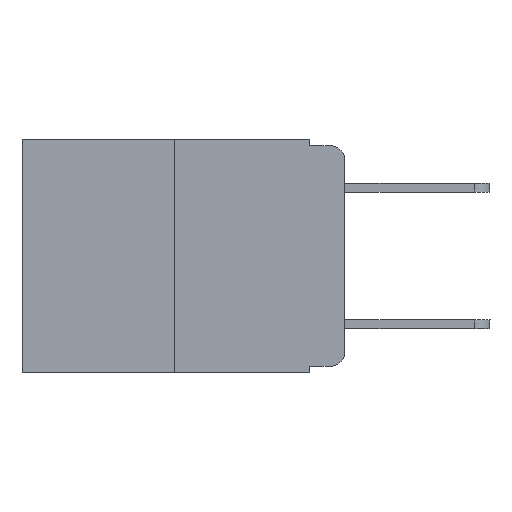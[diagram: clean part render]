
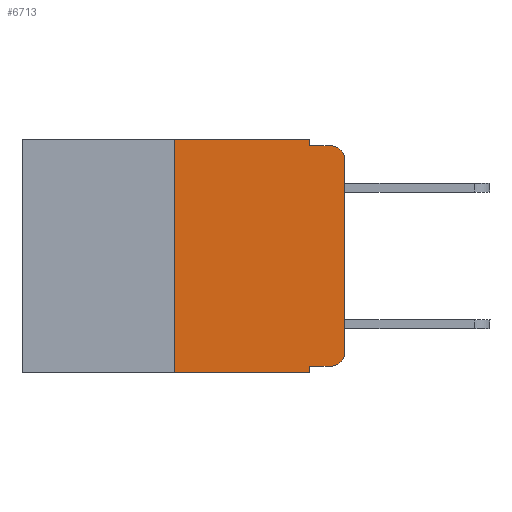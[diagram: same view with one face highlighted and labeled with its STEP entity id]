
A CAD part, left-side view. The second image highlights one B-rep face of the part: STEP entity #6713.
In plain terms, the highlighted planar face has unit normal (-1, 0, 0).
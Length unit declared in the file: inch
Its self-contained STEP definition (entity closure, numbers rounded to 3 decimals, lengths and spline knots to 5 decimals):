
#71 = CARTESIAN_POINT ( 'NONE',  ( 0., 0.051, -0.343 ) ) ;
#630 = VECTOR ( 'NONE', #10684, 39.37008 ) ;
#788 = LINE ( 'NONE', #16542, #19257 ) ;
#1191 = CARTESIAN_POINT ( 'NONE',  ( 0., 0.051, -0.333 ) ) ;
#1439 = EDGE_CURVE ( 'NONE', #18418, #3202, #11320, .T. ) ;
#2270 = VECTOR ( 'NONE', #10813, 39.37008 ) ;
#2386 = AXIS2_PLACEMENT_3D ( 'NONE', #9426, #15730, #13343 ) ;
#3202 = VERTEX_POINT ( 'NONE', #18172 ) ;
#3826 = ORIENTED_EDGE ( 'NONE', *, *, #18937, .F. ) ;
#4298 = CARTESIAN_POINT ( 'NONE',  ( 0., 0.473, 0. ) ) ;
#4370 = LINE ( 'NONE', #7563, #15542 ) ;
#4573 = EDGE_CURVE ( 'NONE', #18636, #16786, #20129, .T. ) ;
#4710 = EDGE_CURVE ( 'NONE', #7278, #18636, #17013, .T. ) ;
#5203 = ORIENTED_EDGE ( 'NONE', *, *, #12139, .F. ) ;
#5859 = DIRECTION ( 'NONE',  ( 0., 0., 1. ) ) ;
#6403 = DIRECTION ( 'NONE',  ( 0., 0., -1. ) ) ;
#6502 = CARTESIAN_POINT ( 'NONE',  ( 0., 0.051, 0. ) ) ;
#6581 = VECTOR ( 'NONE', #14652, 39.37008 ) ;
#6713 = ADVANCED_FACE ( 'NONE', ( #18058 ), #13406, .F. ) ;
#7006 = CARTESIAN_POINT ( 'NONE',  ( 0., 0.051, -0.01 ) ) ;
#7278 = VERTEX_POINT ( 'NONE', #19424 ) ;
#7444 = ORIENTED_EDGE ( 'NONE', *, *, #20322, .F. ) ;
#7563 = CARTESIAN_POINT ( 'NONE',  ( 0., 0.051, -0.333 ) ) ;
#7661 = CARTESIAN_POINT ( 'NONE',  ( 0., 0.02, -0.333 ) ) ;
#7866 = LINE ( 'NONE', #20189, #8780 ) ;
#7986 = CIRCLE ( 'NONE', #18227, 0.02 ) ;
#8211 = CARTESIAN_POINT ( 'NONE',  ( 0., 0., -0.03 ) ) ;
#8314 = EDGE_CURVE ( 'NONE', #15912, #20407, #7986, .T. ) ;
#8780 = VECTOR ( 'NONE', #20401, 39.37008 ) ;
#9102 = ORIENTED_EDGE ( 'NONE', *, *, #8314, .T. ) ;
#9426 = CARTESIAN_POINT ( 'NONE',  ( 0., 0.02, -0.313 ) ) ;
#9769 = DIRECTION ( 'NONE',  ( -1., 0., 0. ) ) ;
#10143 = CARTESIAN_POINT ( 'NONE',  ( 0., 0.25, 0. ) ) ;
#10561 = DIRECTION ( 'NONE',  ( 0., 0., -1. ) ) ;
#10659 = VECTOR ( 'NONE', #6403, 39.37008 ) ;
#10684 = DIRECTION ( 'NONE',  ( 0., 0., 1. ) ) ;
#10779 = ORIENTED_EDGE ( 'NONE', *, *, #16261, .T. ) ;
#10813 = DIRECTION ( 'NONE',  ( 0., -1., 0. ) ) ;
#10919 = LINE ( 'NONE', #12371, #14381 ) ;
#11187 = DIRECTION ( 'NONE',  ( 0., 0., -1. ) ) ;
#11320 = CIRCLE ( 'NONE', #2386, 0.02 ) ;
#11472 = CARTESIAN_POINT ( 'NONE',  ( 0., 0.051, 0. ) ) ;
#11646 = CARTESIAN_POINT ( 'NONE',  ( 0., 0.473, -0.343 ) ) ;
#11724 = EDGE_CURVE ( 'NONE', #3202, #15912, #10919, .T. ) ;
#12035 = ORIENTED_EDGE ( 'NONE', *, *, #11724, .T. ) ;
#12118 = CARTESIAN_POINT ( 'NONE',  ( 0., 0.473, 0. ) ) ;
#12139 = EDGE_CURVE ( 'NONE', #12872, #20407, #7866, .T. ) ;
#12371 = CARTESIAN_POINT ( 'NONE',  ( 0., 0., 0. ) ) ;
#12872 = VERTEX_POINT ( 'NONE', #7006 ) ;
#12929 = AXIS2_PLACEMENT_3D ( 'NONE', #12118, #18432, #10561 ) ;
#12996 = ORIENTED_EDGE ( 'NONE', *, *, #4573, .F. ) ;
#13343 = DIRECTION ( 'NONE',  ( 0., 0., -1. ) ) ;
#13406 = PLANE ( 'NONE',  #12929 ) ;
#13459 = VERTEX_POINT ( 'NONE', #71 ) ;
#14166 = LINE ( 'NONE', #6502, #10659 ) ;
#14179 = EDGE_CURVE ( 'NONE', #7278, #13459, #14449, .T. ) ;
#14381 = VECTOR ( 'NONE', #5859, 39.37008 ) ;
#14426 = CARTESIAN_POINT ( 'NONE',  ( 0., 0.02, -0.03 ) ) ;
#14449 = LINE ( 'NONE', #11646, #6581 ) ;
#14652 = DIRECTION ( 'NONE',  ( 0., -1., 0. ) ) ;
#14789 = EDGE_LOOP ( 'NONE', ( #12035, #9102, #5203, #3826, #12996, #17294, #18212, #7444, #10779, #15254 ) ) ;
#15254 = ORIENTED_EDGE ( 'NONE', *, *, #1439, .T. ) ;
#15542 = VECTOR ( 'NONE', #20201, 39.37008 ) ;
#15730 = DIRECTION ( 'NONE',  ( -1., 0., 0. ) ) ;
#15753 = CARTESIAN_POINT ( 'NONE',  ( 0., 0.25, 0. ) ) ;
#15912 = VERTEX_POINT ( 'NONE', #8211 ) ;
#16077 = DIRECTION ( 'NONE',  ( 0., 0., -1. ) ) ;
#16261 = EDGE_CURVE ( 'NONE', #17124, #18418, #4370, .T. ) ;
#16542 = CARTESIAN_POINT ( 'NONE',  ( 0., 0.051, 0. ) ) ;
#16786 = VERTEX_POINT ( 'NONE', #11472 ) ;
#17013 = LINE ( 'NONE', #15753, #630 ) ;
#17124 = VERTEX_POINT ( 'NONE', #1191 ) ;
#17294 = ORIENTED_EDGE ( 'NONE', *, *, #4710, .F. ) ;
#17406 = CARTESIAN_POINT ( 'NONE',  ( 0., 0.02, -0.01 ) ) ;
#18058 = FACE_OUTER_BOUND ( 'NONE', #14789, .T. ) ;
#18172 = CARTESIAN_POINT ( 'NONE',  ( 0., 0., -0.313 ) ) ;
#18212 = ORIENTED_EDGE ( 'NONE', *, *, #14179, .T. ) ;
#18227 = AXIS2_PLACEMENT_3D ( 'NONE', #14426, #9769, #16077 ) ;
#18418 = VERTEX_POINT ( 'NONE', #7661 ) ;
#18432 = DIRECTION ( 'NONE',  ( 1., 0., 0. ) ) ;
#18636 = VERTEX_POINT ( 'NONE', #10143 ) ;
#18937 = EDGE_CURVE ( 'NONE', #16786, #12872, #14166, .T. ) ;
#19257 = VECTOR ( 'NONE', #11187, 39.37008 ) ;
#19424 = CARTESIAN_POINT ( 'NONE',  ( 0., 0.25, -0.343 ) ) ;
#20129 = LINE ( 'NONE', #4298, #2270 ) ;
#20189 = CARTESIAN_POINT ( 'NONE',  ( 0., 0.051, -0.01 ) ) ;
#20201 = DIRECTION ( 'NONE',  ( 0., -1., 0. ) ) ;
#20322 = EDGE_CURVE ( 'NONE', #17124, #13459, #788, .T. ) ;
#20401 = DIRECTION ( 'NONE',  ( 0., -1., 0. ) ) ;
#20407 = VERTEX_POINT ( 'NONE', #17406 ) ;
